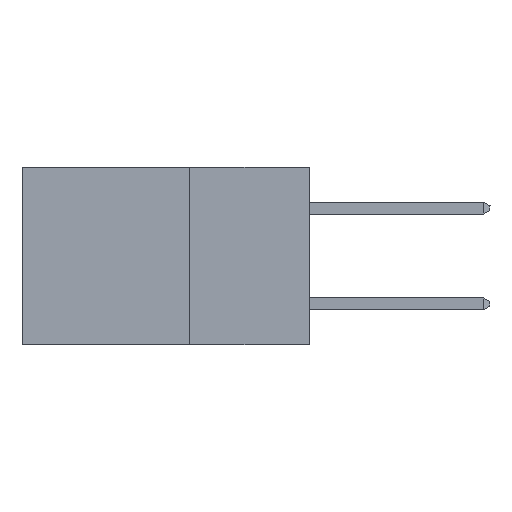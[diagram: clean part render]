
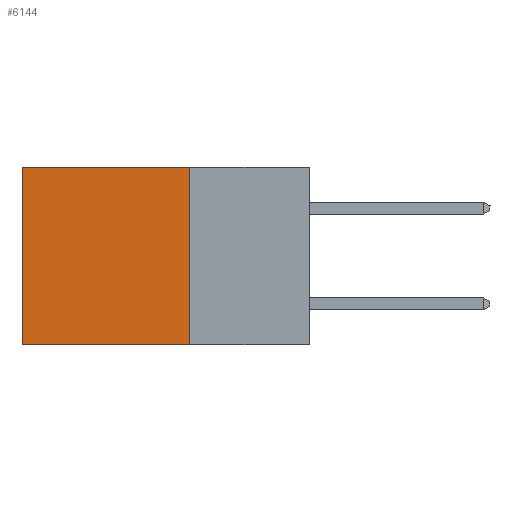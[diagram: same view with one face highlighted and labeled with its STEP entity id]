
A CAD part, left-side view. The second image highlights one B-rep face of the part: STEP entity #6144.
In plain terms, the highlighted planar face has unit normal (-1, 0, 0).
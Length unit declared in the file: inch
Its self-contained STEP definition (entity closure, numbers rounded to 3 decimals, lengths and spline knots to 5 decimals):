
#297 = PLANE ( 'NONE',  #14960 ) ;
#2359 = VERTEX_POINT ( 'NONE', #9082 ) ;
#2878 = DIRECTION ( 'NONE',  ( 0., 0., -1. ) ) ;
#3014 = DIRECTION ( 'NONE',  ( 1., 0., 0. ) ) ;
#3366 = CARTESIAN_POINT ( 'NONE',  ( 0.2875, 0.25, -0.37 ) ) ;
#3513 = ORIENTED_EDGE ( 'NONE', *, *, #11345, .F. ) ;
#4159 = VERTEX_POINT ( 'NONE', #13415 ) ;
#5091 = ORIENTED_EDGE ( 'NONE', *, *, #10076, .T. ) ;
#5529 = CARTESIAN_POINT ( 'NONE',  ( 0.2875, 0.25, -0.37 ) ) ;
#6057 = DIRECTION ( 'NONE',  ( 0., 1., 0. ) ) ;
#6096 = FACE_OUTER_BOUND ( 'NONE', #14995, .T. ) ;
#6144 = ADVANCED_FACE ( 'NONE', ( #6096 ), #297, .F. ) ;
#6378 = CARTESIAN_POINT ( 'NONE',  ( 0.2875, 0.6, 0. ) ) ;
#6487 = CARTESIAN_POINT ( 'NONE',  ( 0.2875, 0.25, 0. ) ) ;
#7187 = VERTEX_POINT ( 'NONE', #3366 ) ;
#7320 = CARTESIAN_POINT ( 'NONE',  ( 0.2875, 0.25, 0. ) ) ;
#7579 = ORIENTED_EDGE ( 'NONE', *, *, #17760, .F. ) ;
#7772 = LINE ( 'NONE', #6378, #14502 ) ;
#8210 = VERTEX_POINT ( 'NONE', #6487 ) ;
#8967 = LINE ( 'NONE', #17714, #15416 ) ;
#9082 = CARTESIAN_POINT ( 'NONE',  ( 0.2875, 0.6, -0.37 ) ) ;
#10076 = EDGE_CURVE ( 'NONE', #4159, #2359, #7772, .T. ) ;
#10642 = ORIENTED_EDGE ( 'NONE', *, *, #12765, .T. ) ;
#11293 = LINE ( 'NONE', #14078, #15419 ) ;
#11345 = EDGE_CURVE ( 'NONE', #8210, #7187, #11293, .T. ) ;
#11788 = DIRECTION ( 'NONE',  ( 0., 0., -1. ) ) ;
#12520 = DIRECTION ( 'NONE',  ( 0., 0., -1. ) ) ;
#12765 = EDGE_CURVE ( 'NONE', #8210, #4159, #8967, .T. ) ;
#13415 = CARTESIAN_POINT ( 'NONE',  ( 0.2875, 0.6, 0. ) ) ;
#13756 = VECTOR ( 'NONE', #17005, 39.37008 ) ;
#14078 = CARTESIAN_POINT ( 'NONE',  ( 0.2875, 0.25, 0. ) ) ;
#14502 = VECTOR ( 'NONE', #12520, 39.37008 ) ;
#14960 = AXIS2_PLACEMENT_3D ( 'NONE', #7320, #3014, #11788 ) ;
#14995 = EDGE_LOOP ( 'NONE', ( #5091, #7579, #3513, #10642 ) ) ;
#15416 = VECTOR ( 'NONE', #6057, 39.37008 ) ;
#15419 = VECTOR ( 'NONE', #2878, 39.37008 ) ;
#17005 = DIRECTION ( 'NONE',  ( 0., 1., 0. ) ) ;
#17105 = LINE ( 'NONE', #5529, #13756 ) ;
#17714 = CARTESIAN_POINT ( 'NONE',  ( 0.2875, 0.25, 0. ) ) ;
#17760 = EDGE_CURVE ( 'NONE', #7187, #2359, #17105, .T. ) ;
